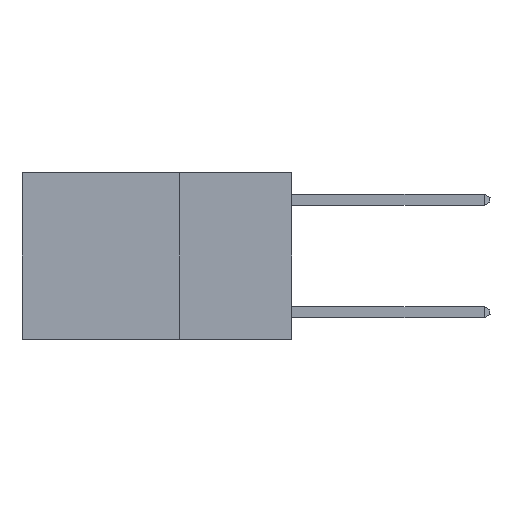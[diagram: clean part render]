
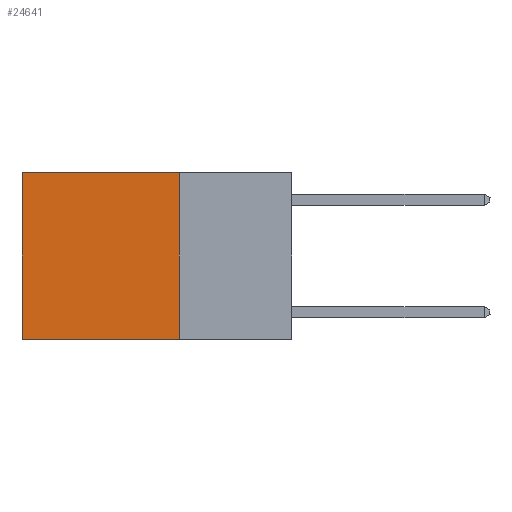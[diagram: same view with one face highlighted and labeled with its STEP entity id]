
A CAD part, left-side view. The second image highlights one B-rep face of the part: STEP entity #24641.
In plain terms, the highlighted planar face has unit normal (-1, 0, 0).
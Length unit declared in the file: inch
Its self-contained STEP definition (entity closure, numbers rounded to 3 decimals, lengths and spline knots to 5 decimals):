
#70 = VERTEX_POINT ( 'NONE', #18658 ) ;
#199 = CARTESIAN_POINT ( 'NONE',  ( 0.2625, 0.25, 0. ) ) ;
#430 = DIRECTION ( 'NONE',  ( 0., 1., 0. ) ) ;
#1501 = EDGE_CURVE ( 'NONE', #70, #18105, #28536, .T. ) ;
#1563 = EDGE_CURVE ( 'NONE', #26399, #18105, #9884, .T. ) ;
#2351 = CARTESIAN_POINT ( 'NONE',  ( 0.2625, 0.6, 0. ) ) ;
#2360 = EDGE_LOOP ( 'NONE', ( #11147, #20094, #13812, #18906 ) ) ;
#2789 = DIRECTION ( 'NONE',  ( 0., 0., -1. ) ) ;
#3427 = VECTOR ( 'NONE', #21555, 39.37008 ) ;
#4996 = CARTESIAN_POINT ( 'NONE',  ( 0.2625, 0.25, -0.37 ) ) ;
#6024 = CARTESIAN_POINT ( 'NONE',  ( 0.2625, 0.25, 0. ) ) ;
#6129 = VERTEX_POINT ( 'NONE', #21545 ) ;
#6337 = DIRECTION ( 'NONE',  ( 1., 0., 0. ) ) ;
#8774 = VECTOR ( 'NONE', #430, 39.37008 ) ;
#9086 = VECTOR ( 'NONE', #19886, 39.37008 ) ;
#9884 = LINE ( 'NONE', #23985, #26315 ) ;
#11147 = ORIENTED_EDGE ( 'NONE', *, *, #1563, .T. ) ;
#11200 = DIRECTION ( 'NONE',  ( 0., 0., -1. ) ) ;
#13092 = PLANE ( 'NONE',  #24579 ) ;
#13716 = CARTESIAN_POINT ( 'NONE',  ( 0.2625, 0.25, 0. ) ) ;
#13812 = ORIENTED_EDGE ( 'NONE', *, *, #22417, .F. ) ;
#18105 = VERTEX_POINT ( 'NONE', #21459 ) ;
#18658 = CARTESIAN_POINT ( 'NONE',  ( 0.2625, 0.25, -0.37 ) ) ;
#18906 = ORIENTED_EDGE ( 'NONE', *, *, #25851, .T. ) ;
#19886 = DIRECTION ( 'NONE',  ( 0., 1., 0. ) ) ;
#20094 = ORIENTED_EDGE ( 'NONE', *, *, #1501, .F. ) ;
#20458 = LINE ( 'NONE', #6024, #9086 ) ;
#21459 = CARTESIAN_POINT ( 'NONE',  ( 0.2625, 0.6, -0.37 ) ) ;
#21545 = CARTESIAN_POINT ( 'NONE',  ( 0.2625, 0.25, 0. ) ) ;
#21555 = DIRECTION ( 'NONE',  ( 0., 0., -1. ) ) ;
#22417 = EDGE_CURVE ( 'NONE', #6129, #70, #26415, .T. ) ;
#23985 = CARTESIAN_POINT ( 'NONE',  ( 0.2625, 0.6, 0. ) ) ;
#24579 = AXIS2_PLACEMENT_3D ( 'NONE', #13716, #6337, #11200 ) ;
#24641 = ADVANCED_FACE ( 'NONE', ( #29860 ), #13092, .F. ) ;
#25851 = EDGE_CURVE ( 'NONE', #6129, #26399, #20458, .T. ) ;
#26315 = VECTOR ( 'NONE', #2789, 39.37008 ) ;
#26399 = VERTEX_POINT ( 'NONE', #2351 ) ;
#26415 = LINE ( 'NONE', #199, #3427 ) ;
#28536 = LINE ( 'NONE', #4996, #8774 ) ;
#29860 = FACE_OUTER_BOUND ( 'NONE', #2360, .T. ) ;
